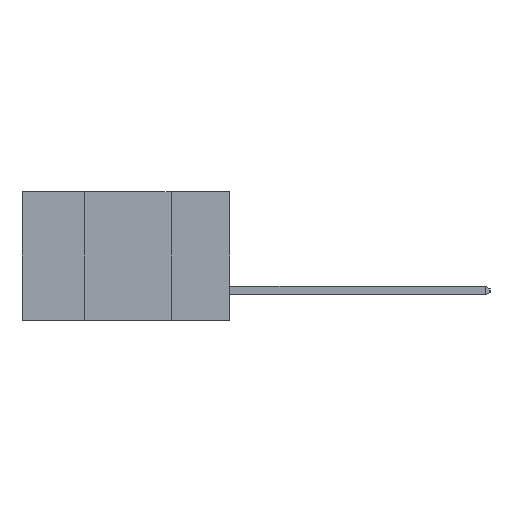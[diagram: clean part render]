
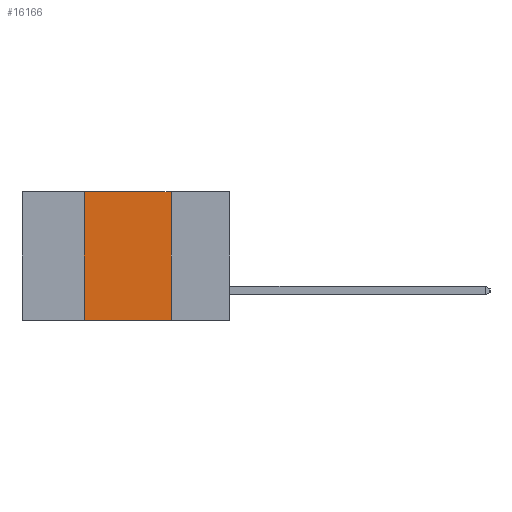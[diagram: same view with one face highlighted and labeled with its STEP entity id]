
A CAD part, left-side view. The second image highlights one B-rep face of the part: STEP entity #16166.
In plain terms, the highlighted planar face has unit normal (-1, 0, 0).
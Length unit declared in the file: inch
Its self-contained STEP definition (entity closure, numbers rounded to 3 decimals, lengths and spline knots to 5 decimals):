
#397 = ORIENTED_EDGE ( 'NONE', *, *, #25128, .T. ) ;
#1836 = DIRECTION ( 'NONE',  ( 0., -1., 0. ) ) ;
#3662 = LINE ( 'NONE', #29197, #23304 ) ;
#4236 = DIRECTION ( 'NONE',  ( 0., 0., -1. ) ) ;
#5067 = FACE_OUTER_BOUND ( 'NONE', #21033, .T. ) ;
#6265 = EDGE_CURVE ( 'NONE', #21004, #6630, #17367, .T. ) ;
#6291 = VERTEX_POINT ( 'NONE', #28233 ) ;
#6295 = CARTESIAN_POINT ( 'NONE',  ( 0., 0.42, -0.37 ) ) ;
#6630 = VERTEX_POINT ( 'NONE', #30874 ) ;
#7179 = DIRECTION ( 'NONE',  ( 0., 0., 1. ) ) ;
#9320 = CARTESIAN_POINT ( 'NONE',  ( 0., 0.17, 0. ) ) ;
#9844 = EDGE_CURVE ( 'NONE', #17651, #21004, #3662, .T. ) ;
#10333 = VECTOR ( 'NONE', #1836, 39.37008 ) ;
#10482 = PLANE ( 'NONE',  #23048 ) ;
#10585 = CARTESIAN_POINT ( 'NONE',  ( 0., 0.6, 0. ) ) ;
#13030 = DIRECTION ( 'NONE',  ( 0., 0., -1. ) ) ;
#13335 = VECTOR ( 'NONE', #4236, 39.37008 ) ;
#16166 = ADVANCED_FACE ( 'NONE', ( #5067 ), #10482, .F. ) ;
#16816 = LINE ( 'NONE', #23959, #10333 ) ;
#17367 = LINE ( 'NONE', #26976, #28697 ) ;
#17651 = VERTEX_POINT ( 'NONE', #6295 ) ;
#17891 = ORIENTED_EDGE ( 'NONE', *, *, #19656, .F. ) ;
#19414 = ORIENTED_EDGE ( 'NONE', *, *, #9844, .F. ) ;
#19656 = EDGE_CURVE ( 'NONE', #6630, #6291, #27018, .T. ) ;
#21004 = VERTEX_POINT ( 'NONE', #26794 ) ;
#21033 = EDGE_LOOP ( 'NONE', ( #17891, #30725, #19414, #397 ) ) ;
#23048 = AXIS2_PLACEMENT_3D ( 'NONE', #10585, #27559, #13030 ) ;
#23304 = VECTOR ( 'NONE', #7179, 39.37008 ) ;
#23959 = CARTESIAN_POINT ( 'NONE',  ( 0., 0.6, -0.37 ) ) ;
#25128 = EDGE_CURVE ( 'NONE', #17651, #6291, #16816, .T. ) ;
#26794 = CARTESIAN_POINT ( 'NONE',  ( 0., 0.42, 0. ) ) ;
#26976 = CARTESIAN_POINT ( 'NONE',  ( 0., 0.6, 0. ) ) ;
#27018 = LINE ( 'NONE', #9320, #13335 ) ;
#27158 = DIRECTION ( 'NONE',  ( 0., -1., 0. ) ) ;
#27559 = DIRECTION ( 'NONE',  ( 1., 0., 0. ) ) ;
#28233 = CARTESIAN_POINT ( 'NONE',  ( 0., 0.17, -0.37 ) ) ;
#28697 = VECTOR ( 'NONE', #27158, 39.37008 ) ;
#29197 = CARTESIAN_POINT ( 'NONE',  ( 0., 0.42, 0. ) ) ;
#30725 = ORIENTED_EDGE ( 'NONE', *, *, #6265, .F. ) ;
#30874 = CARTESIAN_POINT ( 'NONE',  ( 0., 0.17, 0. ) ) ;
